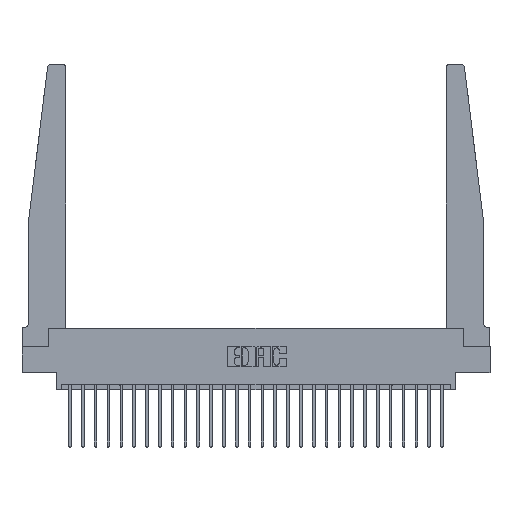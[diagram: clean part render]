
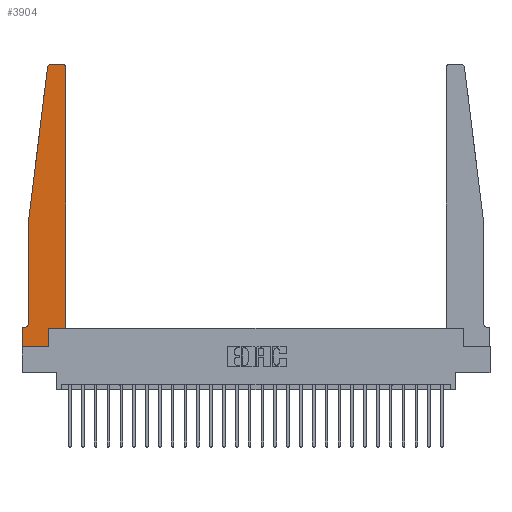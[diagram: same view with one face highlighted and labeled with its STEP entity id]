
A CAD part, top view. The second image highlights one B-rep face of the part: STEP entity #3904.
In plain terms, the highlighted planar face has unit normal (0, 0, 1).
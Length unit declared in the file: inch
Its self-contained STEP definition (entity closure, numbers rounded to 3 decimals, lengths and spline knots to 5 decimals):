
#63 = LINE ( 'NONE', #12751, #25640 ) ;
#224 = CARTESIAN_POINT ( 'NONE',  ( 0.2605, 0.18, 0.37 ) ) ;
#291 = EDGE_CURVE ( 'NONE', #12692, #21680, #11310, .T. ) ;
#1434 = CIRCLE ( 'NONE', #5650, 0.05 ) ;
#1724 = VECTOR ( 'NONE', #23258, 39.37008 ) ;
#1880 = DIRECTION ( 'NONE',  ( 0., 0., 1. ) ) ;
#1962 = LINE ( 'NONE', #12309, #12086 ) ;
#2435 = AXIS2_PLACEMENT_3D ( 'NONE', #16689, #4548, #18751 ) ;
#2587 = DIRECTION ( 'NONE',  ( -1., 0., 0. ) ) ;
#2722 = EDGE_CURVE ( 'NONE', #21680, #2914, #17898, .T. ) ;
#2914 = VERTEX_POINT ( 'NONE', #5528 ) ;
#3123 = DIRECTION ( 'NONE',  ( 1., 0., 0. ) ) ;
#3532 = CARTESIAN_POINT ( 'NONE',  ( 0.065, 1.25, 0.37 ) ) ;
#3541 = ORIENTED_EDGE ( 'NONE', *, *, #291, .T. ) ;
#3833 = VERTEX_POINT ( 'NONE', #13734 ) ;
#3904 = ADVANCED_FACE ( 'NONE', ( #19867 ), #13994, .T. ) ;
#4060 = CARTESIAN_POINT ( 'NONE',  ( 0.24675, 2.72367, 0.37 ) ) ;
#4310 = VECTOR ( 'NONE', #15830, 39.37008 ) ;
#4548 = DIRECTION ( 'NONE',  ( 0., 0., 1. ) ) ;
#5528 = CARTESIAN_POINT ( 'NONE',  ( 0., 0., 0.37 ) ) ;
#5536 = CARTESIAN_POINT ( 'NONE',  ( 0.015, 0.2375, 0.37 ) ) ;
#5545 = EDGE_CURVE ( 'NONE', #2914, #25948, #26017, .T. ) ;
#5650 = AXIS2_PLACEMENT_3D ( 'NONE', #5536, #19735, #7576 ) ;
#6251 = ORIENTED_EDGE ( 'NONE', *, *, #22557, .T. ) ;
#6345 = CARTESIAN_POINT ( 'NONE',  ( 0.27653, 2.72, 0.37 ) ) ;
#6523 = LINE ( 'NONE', #9330, #22054 ) ;
#7576 = DIRECTION ( 'NONE',  ( -1., 0., 0. ) ) ;
#7587 = CIRCLE ( 'NONE', #2435, 0.03 ) ;
#7755 = VERTEX_POINT ( 'NONE', #23640 ) ;
#8080 = VERTEX_POINT ( 'NONE', #24730 ) ;
#8364 = DIRECTION ( 'NONE',  ( 1., 0., 0. ) ) ;
#8752 = CIRCLE ( 'NONE', #22488, 0.03 ) ;
#9011 = AXIS2_PLACEMENT_3D ( 'NONE', #18019, #1880, #16040 ) ;
#9265 = VECTOR ( 'NONE', #10309, 39.37008 ) ;
#9330 = CARTESIAN_POINT ( 'NONE',  ( 0.425, 0.18, 0.37 ) ) ;
#9530 = CARTESIAN_POINT ( 'NONE',  ( 0.425, 2.72, 0.37 ) ) ;
#10309 = DIRECTION ( 'NONE',  ( 0., 1., 0. ) ) ;
#11310 = LINE ( 'NONE', #25005, #26120 ) ;
#11368 = DIRECTION ( 'NONE',  ( 1., 0., 0. ) ) ;
#11477 = ORIENTED_EDGE ( 'NONE', *, *, #5545, .T. ) ;
#11758 = ORIENTED_EDGE ( 'NONE', *, *, #15054, .T. ) ;
#11887 = EDGE_CURVE ( 'NONE', #21125, #12960, #1962, .T. ) ;
#12086 = VECTOR ( 'NONE', #24415, 39.37008 ) ;
#12309 = CARTESIAN_POINT ( 'NONE',  ( 0.065, 1.25, 0.37 ) ) ;
#12472 = DIRECTION ( 'NONE',  ( -1., 0., 0. ) ) ;
#12579 = LINE ( 'NONE', #18346, #22741 ) ;
#12609 = VERTEX_POINT ( 'NONE', #18371 ) ;
#12692 = VERTEX_POINT ( 'NONE', #16569 ) ;
#12751 = CARTESIAN_POINT ( 'NONE',  ( 0.25, 2.75, 0.37 ) ) ;
#12815 = ORIENTED_EDGE ( 'NONE', *, *, #2722, .T. ) ;
#12960 = VERTEX_POINT ( 'NONE', #3532 ) ;
#13193 = ORIENTED_EDGE ( 'NONE', *, *, #16785, .T. ) ;
#13203 = EDGE_LOOP ( 'NONE', ( #6251, #19016, #23076, #11758, #13193, #3541, #12815, #11477, #18476, #20892, #20226, #16002 ) ) ;
#13734 = CARTESIAN_POINT ( 'NONE',  ( 0.395, 2.75, 0.37 ) ) ;
#13777 = CARTESIAN_POINT ( 'NONE',  ( 0.425, 0.18, 0.37 ) ) ;
#13994 = PLANE ( 'NONE',  #9011 ) ;
#15054 = EDGE_CURVE ( 'NONE', #12960, #8080, #12579, .T. ) ;
#15082 = LINE ( 'NONE', #13777, #4310 ) ;
#15098 = CARTESIAN_POINT ( 'NONE',  ( 0., 0., 0.37 ) ) ;
#15828 = CARTESIAN_POINT ( 'NONE',  ( 0., 0.1875, 0.37 ) ) ;
#15830 = DIRECTION ( 'NONE',  ( 0., 1., 0. ) ) ;
#16002 = ORIENTED_EDGE ( 'NONE', *, *, #17146, .T. ) ;
#16040 = DIRECTION ( 'NONE',  ( 1., 0., 0. ) ) ;
#16569 = CARTESIAN_POINT ( 'NONE',  ( 0.015, 0.1875, 0.37 ) ) ;
#16689 = CARTESIAN_POINT ( 'NONE',  ( 0.395, 2.72, 0.37 ) ) ;
#16785 = EDGE_CURVE ( 'NONE', #8080, #12692, #1434, .T. ) ;
#17146 = EDGE_CURVE ( 'NONE', #19217, #3833, #7587, .T. ) ;
#17239 = CARTESIAN_POINT ( 'NONE',  ( 0., 0., 0.37 ) ) ;
#17898 = LINE ( 'NONE', #15098, #1724 ) ;
#17907 = CARTESIAN_POINT ( 'NONE',  ( 0.2605, 0.18, 0.37 ) ) ;
#18019 = CARTESIAN_POINT ( 'NONE',  ( 0., 0.1875, 0.37 ) ) ;
#18346 = CARTESIAN_POINT ( 'NONE',  ( 0.065, 1.25, 0.37 ) ) ;
#18371 = CARTESIAN_POINT ( 'NONE',  ( 0.27653, 2.75, 0.37 ) ) ;
#18476 = ORIENTED_EDGE ( 'NONE', *, *, #21901, .T. ) ;
#18751 = DIRECTION ( 'NONE',  ( 1., 0., 0. ) ) ;
#19016 = ORIENTED_EDGE ( 'NONE', *, *, #19497, .T. ) ;
#19217 = VERTEX_POINT ( 'NONE', #9530 ) ;
#19307 = VERTEX_POINT ( 'NONE', #17907 ) ;
#19497 = EDGE_CURVE ( 'NONE', #12609, #21125, #8752, .T. ) ;
#19735 = DIRECTION ( 'NONE',  ( 0., 0., -1. ) ) ;
#19855 = EDGE_CURVE ( 'NONE', #19307, #7755, #6523, .T. ) ;
#19867 = FACE_OUTER_BOUND ( 'NONE', #13203, .T. ) ;
#20078 = LINE ( 'NONE', #224, #9265 ) ;
#20226 = ORIENTED_EDGE ( 'NONE', *, *, #23553, .T. ) ;
#20366 = DIRECTION ( 'NONE',  ( 0., -1., 0. ) ) ;
#20526 = DIRECTION ( 'NONE',  ( 0., 0., 1. ) ) ;
#20721 = VECTOR ( 'NONE', #3123, 39.37008 ) ;
#20892 = ORIENTED_EDGE ( 'NONE', *, *, #19855, .T. ) ;
#21125 = VERTEX_POINT ( 'NONE', #4060 ) ;
#21680 = VERTEX_POINT ( 'NONE', #15828 ) ;
#21901 = EDGE_CURVE ( 'NONE', #25948, #19307, #20078, .T. ) ;
#22054 = VECTOR ( 'NONE', #11368, 39.37008 ) ;
#22365 = CARTESIAN_POINT ( 'NONE',  ( 0.2605, 0., 0.37 ) ) ;
#22488 = AXIS2_PLACEMENT_3D ( 'NONE', #6345, #20526, #8364 ) ;
#22557 = EDGE_CURVE ( 'NONE', #3833, #12609, #63, .T. ) ;
#22741 = VECTOR ( 'NONE', #20366, 39.37008 ) ;
#23076 = ORIENTED_EDGE ( 'NONE', *, *, #11887, .T. ) ;
#23258 = DIRECTION ( 'NONE',  ( 0., -1., 0. ) ) ;
#23553 = EDGE_CURVE ( 'NONE', #7755, #19217, #15082, .T. ) ;
#23640 = CARTESIAN_POINT ( 'NONE',  ( 0.425, 0.18, 0.37 ) ) ;
#24415 = DIRECTION ( 'NONE',  ( -0.122, -0.992, 0. ) ) ;
#24730 = CARTESIAN_POINT ( 'NONE',  ( 0.065, 0.2375, 0.37 ) ) ;
#25005 = CARTESIAN_POINT ( 'NONE',  ( 0.065, 0.1875, 0.37 ) ) ;
#25640 = VECTOR ( 'NONE', #2587, 39.37008 ) ;
#25948 = VERTEX_POINT ( 'NONE', #22365 ) ;
#26017 = LINE ( 'NONE', #17239, #20721 ) ;
#26120 = VECTOR ( 'NONE', #12472, 39.37008 ) ;
